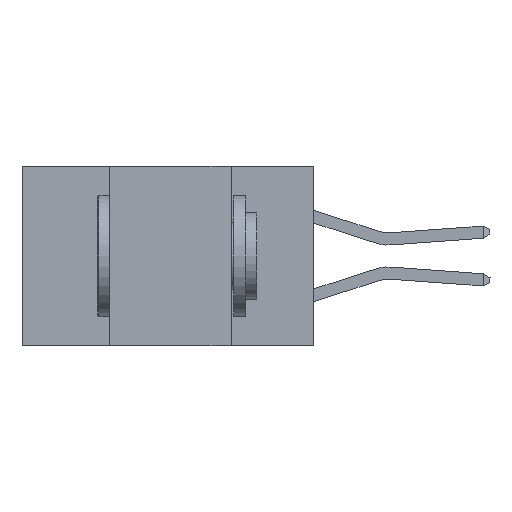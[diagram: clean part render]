
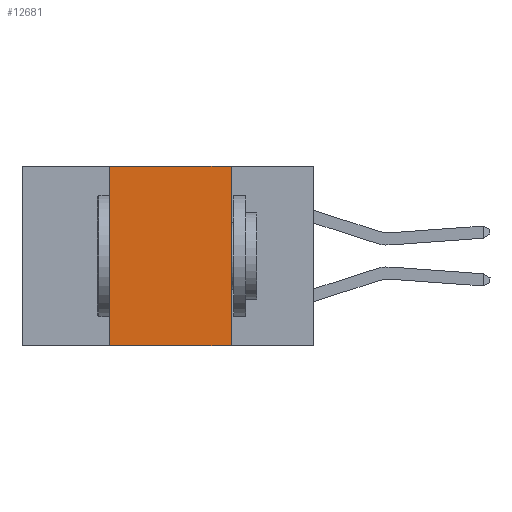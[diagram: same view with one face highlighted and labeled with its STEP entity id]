
A CAD part, left-side view. The second image highlights one B-rep face of the part: STEP entity #12681.
In plain terms, the highlighted planar face has unit normal (-1, 0, 0).
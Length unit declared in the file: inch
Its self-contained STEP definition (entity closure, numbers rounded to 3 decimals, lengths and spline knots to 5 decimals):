
#318 = CARTESIAN_POINT ( 'NONE',  ( 0., 0.42, -0.37 ) ) ;
#624 = CARTESIAN_POINT ( 'NONE',  ( 0., 0.6, -0.37 ) ) ;
#1580 = CARTESIAN_POINT ( 'NONE',  ( 0., 0.17, 0. ) ) ;
#1667 = EDGE_CURVE ( 'NONE', #13517, #2558, #3030, .T. ) ;
#1983 = DIRECTION ( 'NONE',  ( 0., -1., 0. ) ) ;
#2129 = LINE ( 'NONE', #1580, #7206 ) ;
#2558 = VERTEX_POINT ( 'NONE', #9756 ) ;
#2823 = DIRECTION ( 'NONE',  ( 0., 0., -1. ) ) ;
#3030 = LINE ( 'NONE', #624, #10884 ) ;
#3121 = CARTESIAN_POINT ( 'NONE',  ( 0., 0.42, 0. ) ) ;
#3919 = FACE_OUTER_BOUND ( 'NONE', #16926, .T. ) ;
#5667 = DIRECTION ( 'NONE',  ( 0., 0., -1. ) ) ;
#5691 = CARTESIAN_POINT ( 'NONE',  ( 0., 0.6, 0. ) ) ;
#5699 = EDGE_CURVE ( 'NONE', #6392, #6743, #9265, .T. ) ;
#5917 = ORIENTED_EDGE ( 'NONE', *, *, #1667, .T. ) ;
#6392 = VERTEX_POINT ( 'NONE', #3121 ) ;
#6743 = VERTEX_POINT ( 'NONE', #12205 ) ;
#7206 = VECTOR ( 'NONE', #5667, 39.37008 ) ;
#8202 = ORIENTED_EDGE ( 'NONE', *, *, #11960, .F. ) ;
#9105 = DIRECTION ( 'NONE',  ( 0., 0., 1. ) ) ;
#9265 = LINE ( 'NONE', #5691, #9685 ) ;
#9529 = PLANE ( 'NONE',  #11808 ) ;
#9685 = VECTOR ( 'NONE', #15216, 39.37008 ) ;
#9756 = CARTESIAN_POINT ( 'NONE',  ( 0., 0.17, -0.37 ) ) ;
#10783 = CARTESIAN_POINT ( 'NONE',  ( 0., 0.6, 0. ) ) ;
#10884 = VECTOR ( 'NONE', #1983, 39.37008 ) ;
#11808 = AXIS2_PLACEMENT_3D ( 'NONE', #10783, #16329, #2823 ) ;
#11830 = CARTESIAN_POINT ( 'NONE',  ( 0., 0.42, 0. ) ) ;
#11867 = ORIENTED_EDGE ( 'NONE', *, *, #5699, .F. ) ;
#11960 = EDGE_CURVE ( 'NONE', #13517, #6392, #15851, .T. ) ;
#12205 = CARTESIAN_POINT ( 'NONE',  ( 0., 0.17, 0. ) ) ;
#12681 = ADVANCED_FACE ( 'NONE', ( #3919 ), #9529, .F. ) ;
#13517 = VERTEX_POINT ( 'NONE', #318 ) ;
#13546 = ORIENTED_EDGE ( 'NONE', *, *, #15571, .F. ) ;
#14996 = VECTOR ( 'NONE', #9105, 39.37008 ) ;
#15216 = DIRECTION ( 'NONE',  ( 0., -1., 0. ) ) ;
#15571 = EDGE_CURVE ( 'NONE', #6743, #2558, #2129, .T. ) ;
#15851 = LINE ( 'NONE', #11830, #14996 ) ;
#16329 = DIRECTION ( 'NONE',  ( 1., 0., 0. ) ) ;
#16926 = EDGE_LOOP ( 'NONE', ( #13546, #11867, #8202, #5917 ) ) ;
